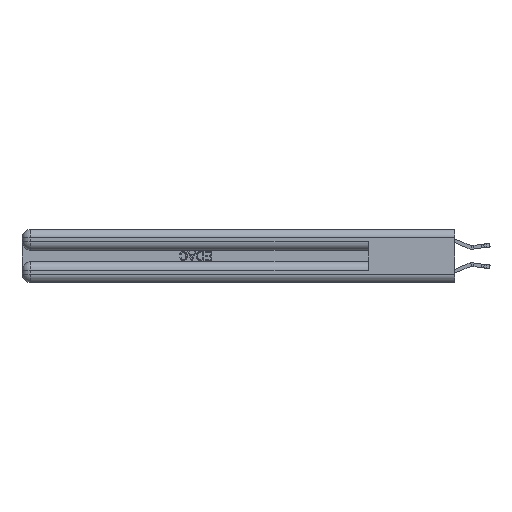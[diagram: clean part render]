
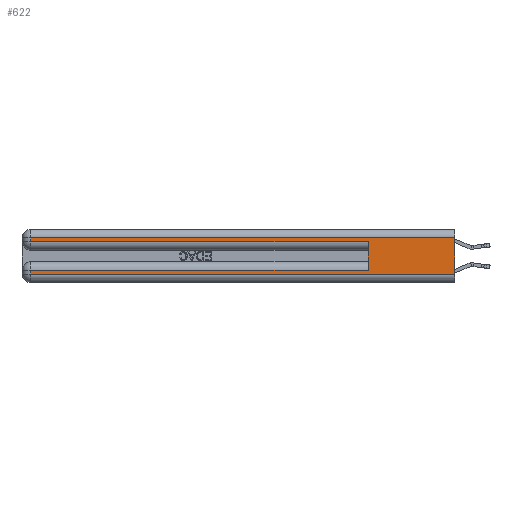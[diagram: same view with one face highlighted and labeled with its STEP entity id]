
A CAD part, left-side view. The second image highlights one B-rep face of the part: STEP entity #622.
In plain terms, the highlighted planar face has unit normal (-1, 0, 0).
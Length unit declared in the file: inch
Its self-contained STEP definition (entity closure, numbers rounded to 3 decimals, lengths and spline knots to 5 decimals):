
#340 = CARTESIAN_POINT ( 'NONE',  ( 0., 0., 0.37 ) ) ;
#622 = ADVANCED_FACE ( 'NONE', ( #19805 ), #24578, .F. ) ;
#737 = VECTOR ( 'NONE', #802, 39.37008 ) ;
#802 = DIRECTION ( 'NONE',  ( 0., 0., -1. ) ) ;
#950 = LINE ( 'NONE', #4261, #24978 ) ;
#1369 = CARTESIAN_POINT ( 'NONE',  ( 0., 2.94, 0.085 ) ) ;
#1401 = CARTESIAN_POINT ( 'NONE',  ( 0., 0., 0.31 ) ) ;
#1551 = CARTESIAN_POINT ( 'NONE',  ( 0., 0., 0.285 ) ) ;
#1915 = ORIENTED_EDGE ( 'NONE', *, *, #14110, .F. ) ;
#3438 = EDGE_CURVE ( 'NONE', #21731, #15048, #21215, .T. ) ;
#3863 = CARTESIAN_POINT ( 'NONE',  ( 0., 2.94, 0.06 ) ) ;
#4261 = CARTESIAN_POINT ( 'NONE',  ( 0., 2.94, 0.37 ) ) ;
#4322 = CARTESIAN_POINT ( 'NONE',  ( 0., 0.6, 0.145 ) ) ;
#5053 = ORIENTED_EDGE ( 'NONE', *, *, #30341, .T. ) ;
#5720 = VERTEX_POINT ( 'NONE', #14417 ) ;
#6496 = ORIENTED_EDGE ( 'NONE', *, *, #32389, .T. ) ;
#7610 = DIRECTION ( 'NONE',  ( 0., 1., 0. ) ) ;
#7776 = CARTESIAN_POINT ( 'NONE',  ( 0., 0., 0.31 ) ) ;
#7883 = VERTEX_POINT ( 'NONE', #3863 ) ;
#8374 = VECTOR ( 'NONE', #13128, 39.37008 ) ;
#8794 = ORIENTED_EDGE ( 'NONE', *, *, #20113, .T. ) ;
#9127 = CARTESIAN_POINT ( 'NONE',  ( 0., 2.94, 0.37 ) ) ;
#9344 = LINE ( 'NONE', #16782, #15191 ) ;
#9811 = LINE ( 'NONE', #26245, #22025 ) ;
#10617 = CARTESIAN_POINT ( 'NONE',  ( 0., 0.6, 0.285 ) ) ;
#11170 = DIRECTION ( 'NONE',  ( 0., 0., -1. ) ) ;
#11385 = VERTEX_POINT ( 'NONE', #19402 ) ;
#12185 = EDGE_CURVE ( 'NONE', #11385, #23522, #13474, .T. ) ;
#13128 = DIRECTION ( 'NONE',  ( 0., 1., 0. ) ) ;
#13474 = LINE ( 'NONE', #29533, #8374 ) ;
#14110 = EDGE_CURVE ( 'NONE', #11385, #21832, #14609, .T. ) ;
#14417 = CARTESIAN_POINT ( 'NONE',  ( 0., 2.94, 0.285 ) ) ;
#14609 = LINE ( 'NONE', #4322, #32640 ) ;
#14970 = EDGE_CURVE ( 'NONE', #21731, #22905, #9344, .T. ) ;
#15048 = VERTEX_POINT ( 'NONE', #26310 ) ;
#15191 = VECTOR ( 'NONE', #27569, 39.37008 ) ;
#15366 = LINE ( 'NONE', #1551, #17960 ) ;
#16782 = CARTESIAN_POINT ( 'NONE',  ( 0., 0., 0.37 ) ) ;
#17902 = ORIENTED_EDGE ( 'NONE', *, *, #3438, .T. ) ;
#17960 = VECTOR ( 'NONE', #28610, 39.37008 ) ;
#19402 = CARTESIAN_POINT ( 'NONE',  ( 0., 0.6, 0.085 ) ) ;
#19565 = LINE ( 'NONE', #9127, #737 ) ;
#19805 = FACE_OUTER_BOUND ( 'NONE', #30298, .T. ) ;
#20113 = EDGE_CURVE ( 'NONE', #23522, #7883, #19565, .T. ) ;
#20868 = AXIS2_PLACEMENT_3D ( 'NONE', #340, #21928, #11170 ) ;
#21188 = EDGE_CURVE ( 'NONE', #15048, #5720, #950, .T. ) ;
#21215 = LINE ( 'NONE', #7776, #27861 ) ;
#21677 = ORIENTED_EDGE ( 'NONE', *, *, #12185, .T. ) ;
#21731 = VERTEX_POINT ( 'NONE', #1401 ) ;
#21832 = VERTEX_POINT ( 'NONE', #10617 ) ;
#21928 = DIRECTION ( 'NONE',  ( 1., 0., 0. ) ) ;
#22025 = VECTOR ( 'NONE', #29067, 39.37008 ) ;
#22266 = ORIENTED_EDGE ( 'NONE', *, *, #14970, .F. ) ;
#22905 = VERTEX_POINT ( 'NONE', #29598 ) ;
#23522 = VERTEX_POINT ( 'NONE', #1369 ) ;
#24578 = PLANE ( 'NONE',  #20868 ) ;
#24978 = VECTOR ( 'NONE', #33964, 39.37008 ) ;
#26245 = CARTESIAN_POINT ( 'NONE',  ( 0., 0., 0.06 ) ) ;
#26310 = CARTESIAN_POINT ( 'NONE',  ( 0., 2.94, 0.31 ) ) ;
#27569 = DIRECTION ( 'NONE',  ( 0., 0., -1. ) ) ;
#27861 = VECTOR ( 'NONE', #7610, 39.37008 ) ;
#28383 = DIRECTION ( 'NONE',  ( 0., 0., 1. ) ) ;
#28610 = DIRECTION ( 'NONE',  ( 0., -1., 0. ) ) ;
#29067 = DIRECTION ( 'NONE',  ( 0., -1., 0. ) ) ;
#29533 = CARTESIAN_POINT ( 'NONE',  ( 0., 0., 0.085 ) ) ;
#29598 = CARTESIAN_POINT ( 'NONE',  ( 0., 0., 0.06 ) ) ;
#30298 = EDGE_LOOP ( 'NONE', ( #22266, #17902, #33348, #5053, #1915, #21677, #8794, #6496 ) ) ;
#30341 = EDGE_CURVE ( 'NONE', #5720, #21832, #15366, .T. ) ;
#32389 = EDGE_CURVE ( 'NONE', #7883, #22905, #9811, .T. ) ;
#32640 = VECTOR ( 'NONE', #28383, 39.37008 ) ;
#33348 = ORIENTED_EDGE ( 'NONE', *, *, #21188, .T. ) ;
#33964 = DIRECTION ( 'NONE',  ( 0., 0., -1. ) ) ;
